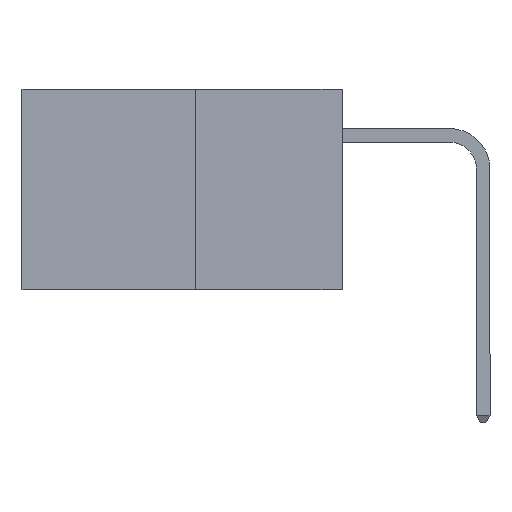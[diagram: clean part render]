
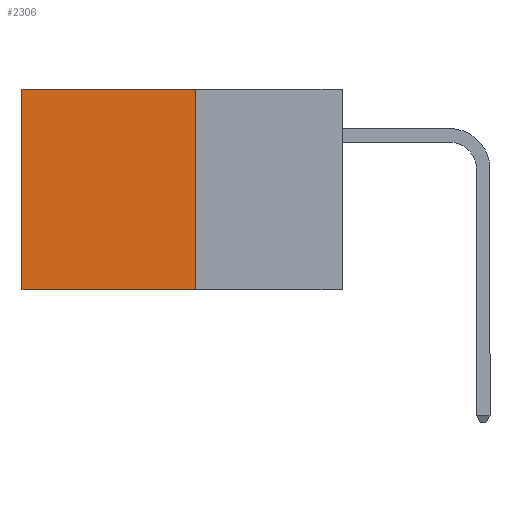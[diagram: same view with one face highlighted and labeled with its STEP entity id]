
A CAD part, left-side view. The second image highlights one B-rep face of the part: STEP entity #2306.
In plain terms, the highlighted planar face has unit normal (-1, 0, 0).
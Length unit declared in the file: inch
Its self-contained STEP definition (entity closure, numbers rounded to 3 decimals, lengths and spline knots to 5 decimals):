
#533 = ORIENTED_EDGE ( 'NONE', *, *, #5543, .T. ) ;
#583 = ORIENTED_EDGE ( 'NONE', *, *, #11296, .F. ) ;
#807 = ORIENTED_EDGE ( 'NONE', *, *, #5667, .F. ) ;
#833 = ORIENTED_EDGE ( 'NONE', *, *, #8431, .T. ) ;
#2198 = CARTESIAN_POINT ( 'NONE',  ( 0.277, 0.27, -0.37 ) ) ;
#2306 = ADVANCED_FACE ( 'NONE', ( #6230 ), #3046, .F. ) ;
#2320 = DIRECTION ( 'NONE',  ( 0., 0., -1. ) ) ;
#2406 = DIRECTION ( 'NONE',  ( 1., 0., 0. ) ) ;
#2907 = VERTEX_POINT ( 'NONE', #6319 ) ;
#3046 = PLANE ( 'NONE',  #4402 ) ;
#3178 = CARTESIAN_POINT ( 'NONE',  ( 0.277, 0.27, -0.37 ) ) ;
#4402 = AXIS2_PLACEMENT_3D ( 'NONE', #3178, #2406, #2320 ) ;
#4682 = VERTEX_POINT ( 'NONE', #7015 ) ;
#5543 = EDGE_CURVE ( 'NONE', #5558, #2907, #11570, .T. ) ;
#5558 = VERTEX_POINT ( 'NONE', #6475 ) ;
#5598 = LINE ( 'NONE', #2198, #10126 ) ;
#5667 = EDGE_CURVE ( 'NONE', #5877, #4682, #8002, .T. ) ;
#5877 = VERTEX_POINT ( 'NONE', #9450 ) ;
#6169 = CARTESIAN_POINT ( 'NONE',  ( 0.277, 0.27, 0. ) ) ;
#6230 = FACE_OUTER_BOUND ( 'NONE', #11618, .T. ) ;
#6259 = DIRECTION ( 'NONE',  ( 0., 1., 0. ) ) ;
#6319 = CARTESIAN_POINT ( 'NONE',  ( 0.277, 0.59, 0. ) ) ;
#6475 = CARTESIAN_POINT ( 'NONE',  ( 0.277, 0.27, 0. ) ) ;
#6600 = CARTESIAN_POINT ( 'NONE',  ( 0.277, 0.27, -0.37 ) ) ;
#6766 = VECTOR ( 'NONE', #6259, 39.37008 ) ;
#7015 = CARTESIAN_POINT ( 'NONE',  ( 0.277, 0.59, -0.37 ) ) ;
#7730 = VECTOR ( 'NONE', #8189, 39.37008 ) ;
#8002 = LINE ( 'NONE', #6600, #7730 ) ;
#8189 = DIRECTION ( 'NONE',  ( 0., 1., 0. ) ) ;
#8238 = LINE ( 'NONE', #9507, #10118 ) ;
#8431 = EDGE_CURVE ( 'NONE', #2907, #4682, #8238, .T. ) ;
#9450 = CARTESIAN_POINT ( 'NONE',  ( 0.277, 0.27, -0.37 ) ) ;
#9507 = CARTESIAN_POINT ( 'NONE',  ( 0.277, 0.59, -0.37 ) ) ;
#10118 = VECTOR ( 'NONE', #10425, 39.37008 ) ;
#10126 = VECTOR ( 'NONE', #11214, 39.37008 ) ;
#10425 = DIRECTION ( 'NONE',  ( 0., 0., -1. ) ) ;
#11214 = DIRECTION ( 'NONE',  ( 0., 0., -1. ) ) ;
#11296 = EDGE_CURVE ( 'NONE', #5558, #5877, #5598, .T. ) ;
#11570 = LINE ( 'NONE', #6169, #6766 ) ;
#11618 = EDGE_LOOP ( 'NONE', ( #833, #807, #583, #533 ) ) ;
